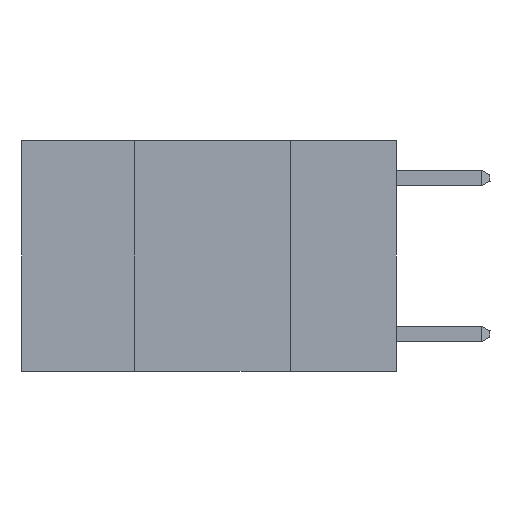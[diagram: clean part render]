
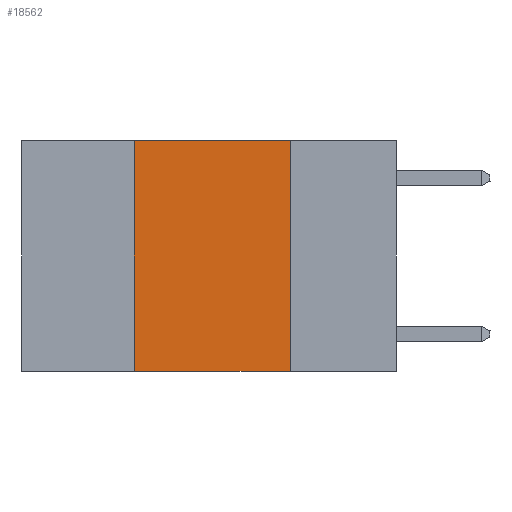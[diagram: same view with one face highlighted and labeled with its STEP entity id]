
A CAD part, left-side view. The second image highlights one B-rep face of the part: STEP entity #18562.
In plain terms, the highlighted planar face has unit normal (-1, 0, 0).
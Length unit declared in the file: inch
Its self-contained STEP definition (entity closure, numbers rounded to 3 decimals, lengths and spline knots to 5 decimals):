
#2262 = VECTOR ( 'NONE', #14119, 39.37008 ) ;
#2566 = VECTOR ( 'NONE', #7060, 39.37008 ) ;
#2836 = VERTEX_POINT ( 'NONE', #10506 ) ;
#2855 = CARTESIAN_POINT ( 'NONE',  ( 0., 0.6, -0.37 ) ) ;
#3163 = DIRECTION ( 'NONE',  ( 0., -1., 0. ) ) ;
#3659 = EDGE_CURVE ( 'NONE', #15102, #2836, #9470, .T. ) ;
#5008 = VECTOR ( 'NONE', #3163, 39.37008 ) ;
#5198 = CARTESIAN_POINT ( 'NONE',  ( 0., 0.42, -0.37 ) ) ;
#6377 = AXIS2_PLACEMENT_3D ( 'NONE', #28072, #13519, #15934 ) ;
#7060 = DIRECTION ( 'NONE',  ( 0., -1., 0. ) ) ;
#9050 = EDGE_LOOP ( 'NONE', ( #10840, #15829, #30705, #30037 ) ) ;
#9347 = EDGE_CURVE ( 'NONE', #10448, #15102, #31058, .T. ) ;
#9470 = LINE ( 'NONE', #28997, #2566 ) ;
#10448 = VERTEX_POINT ( 'NONE', #5198 ) ;
#10474 = CARTESIAN_POINT ( 'NONE',  ( 0., 0.42, 0. ) ) ;
#10506 = CARTESIAN_POINT ( 'NONE',  ( 0., 0.17, 0. ) ) ;
#10840 = ORIENTED_EDGE ( 'NONE', *, *, #17835, .F. ) ;
#11862 = DIRECTION ( 'NONE',  ( 0., 0., 1. ) ) ;
#13519 = DIRECTION ( 'NONE',  ( 1., 0., 0. ) ) ;
#13794 = LINE ( 'NONE', #16216, #2262 ) ;
#14119 = DIRECTION ( 'NONE',  ( 0., 0., -1. ) ) ;
#14613 = VECTOR ( 'NONE', #11862, 39.37008 ) ;
#15102 = VERTEX_POINT ( 'NONE', #10474 ) ;
#15829 = ORIENTED_EDGE ( 'NONE', *, *, #3659, .F. ) ;
#15934 = DIRECTION ( 'NONE',  ( 0., 0., -1. ) ) ;
#16216 = CARTESIAN_POINT ( 'NONE',  ( 0., 0.17, 0. ) ) ;
#17835 = EDGE_CURVE ( 'NONE', #2836, #30242, #13794, .T. ) ;
#18562 = ADVANCED_FACE ( 'NONE', ( #30614 ), #25674, .F. ) ;
#19255 = CARTESIAN_POINT ( 'NONE',  ( 0., 0.42, 0. ) ) ;
#20007 = CARTESIAN_POINT ( 'NONE',  ( 0., 0.17, -0.37 ) ) ;
#20014 = LINE ( 'NONE', #2855, #5008 ) ;
#25674 = PLANE ( 'NONE',  #6377 ) ;
#26960 = EDGE_CURVE ( 'NONE', #10448, #30242, #20014, .T. ) ;
#28072 = CARTESIAN_POINT ( 'NONE',  ( 0., 0.6, 0. ) ) ;
#28997 = CARTESIAN_POINT ( 'NONE',  ( 0., 0.6, 0. ) ) ;
#30037 = ORIENTED_EDGE ( 'NONE', *, *, #26960, .T. ) ;
#30242 = VERTEX_POINT ( 'NONE', #20007 ) ;
#30614 = FACE_OUTER_BOUND ( 'NONE', #9050, .T. ) ;
#30705 = ORIENTED_EDGE ( 'NONE', *, *, #9347, .F. ) ;
#31058 = LINE ( 'NONE', #19255, #14613 ) ;
